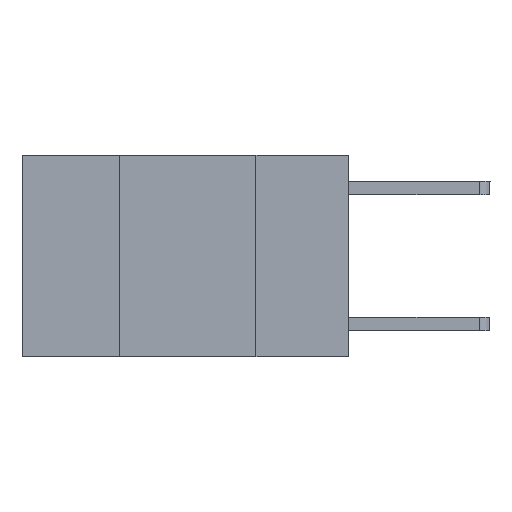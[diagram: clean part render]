
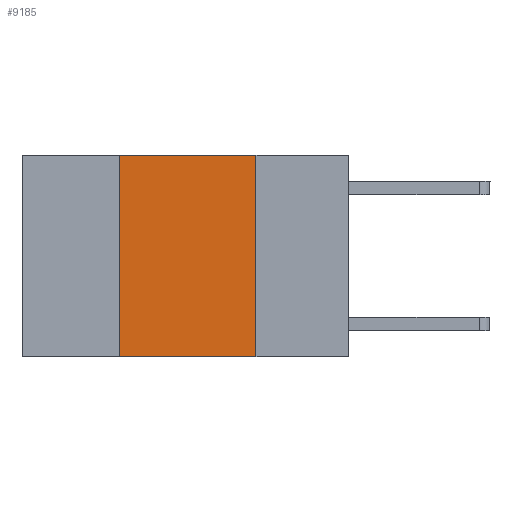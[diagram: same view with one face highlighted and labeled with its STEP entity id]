
A CAD part, left-side view. The second image highlights one B-rep face of the part: STEP entity #9185.
In plain terms, the highlighted planar face has unit normal (-1, 0, 0).
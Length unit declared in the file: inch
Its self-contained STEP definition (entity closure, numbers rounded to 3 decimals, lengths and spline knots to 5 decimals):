
#243 = ORIENTED_EDGE ( 'NONE', *, *, #5395, .T. ) ;
#711 = VERTEX_POINT ( 'NONE', #6536 ) ;
#1129 = AXIS2_PLACEMENT_3D ( 'NONE', #7981, #7186, #8717 ) ;
#1141 = CARTESIAN_POINT ( 'NONE',  ( 0., 0.42, 0. ) ) ;
#1266 = VERTEX_POINT ( 'NONE', #8843 ) ;
#1611 = EDGE_CURVE ( 'NONE', #8305, #2037, #5678, .T. ) ;
#1677 = ORIENTED_EDGE ( 'NONE', *, *, #2086, .F. ) ;
#1894 = PLANE ( 'NONE',  #1129 ) ;
#1995 = DIRECTION ( 'NONE',  ( 0., 0., -1. ) ) ;
#2037 = VERTEX_POINT ( 'NONE', #7048 ) ;
#2086 = EDGE_CURVE ( 'NONE', #2037, #711, #2786, .T. ) ;
#2285 = VECTOR ( 'NONE', #1995, 39.37008 ) ;
#2675 = ORIENTED_EDGE ( 'NONE', *, *, #5130, .F. ) ;
#2786 = LINE ( 'NONE', #8220, #2285 ) ;
#2994 = CARTESIAN_POINT ( 'NONE',  ( 0., 0.6, -0.37 ) ) ;
#4168 = VECTOR ( 'NONE', #5535, 39.37008 ) ;
#4321 = FACE_OUTER_BOUND ( 'NONE', #5861, .T. ) ;
#4834 = CARTESIAN_POINT ( 'NONE',  ( 0., 0.42, 0. ) ) ;
#5130 = EDGE_CURVE ( 'NONE', #1266, #8305, #7014, .T. ) ;
#5322 = LINE ( 'NONE', #2994, #7685 ) ;
#5395 = EDGE_CURVE ( 'NONE', #1266, #711, #5322, .T. ) ;
#5535 = DIRECTION ( 'NONE',  ( 0., 0., 1. ) ) ;
#5678 = LINE ( 'NONE', #5783, #9323 ) ;
#5783 = CARTESIAN_POINT ( 'NONE',  ( 0., 0.6, 0. ) ) ;
#5861 = EDGE_LOOP ( 'NONE', ( #1677, #7759, #2675, #243 ) ) ;
#6536 = CARTESIAN_POINT ( 'NONE',  ( 0., 0.17, -0.37 ) ) ;
#7014 = LINE ( 'NONE', #4834, #4168 ) ;
#7048 = CARTESIAN_POINT ( 'NONE',  ( 0., 0.17, 0. ) ) ;
#7186 = DIRECTION ( 'NONE',  ( 1., 0., 0. ) ) ;
#7685 = VECTOR ( 'NONE', #8191, 39.37008 ) ;
#7759 = ORIENTED_EDGE ( 'NONE', *, *, #1611, .F. ) ;
#7981 = CARTESIAN_POINT ( 'NONE',  ( 0., 0.6, 0. ) ) ;
#8191 = DIRECTION ( 'NONE',  ( 0., -1., 0. ) ) ;
#8220 = CARTESIAN_POINT ( 'NONE',  ( 0., 0.17, 0. ) ) ;
#8305 = VERTEX_POINT ( 'NONE', #1141 ) ;
#8717 = DIRECTION ( 'NONE',  ( 0., 0., -1. ) ) ;
#8781 = DIRECTION ( 'NONE',  ( 0., -1., 0. ) ) ;
#8843 = CARTESIAN_POINT ( 'NONE',  ( 0., 0.42, -0.37 ) ) ;
#9185 = ADVANCED_FACE ( 'NONE', ( #4321 ), #1894, .F. ) ;
#9323 = VECTOR ( 'NONE', #8781, 39.37008 ) ;
